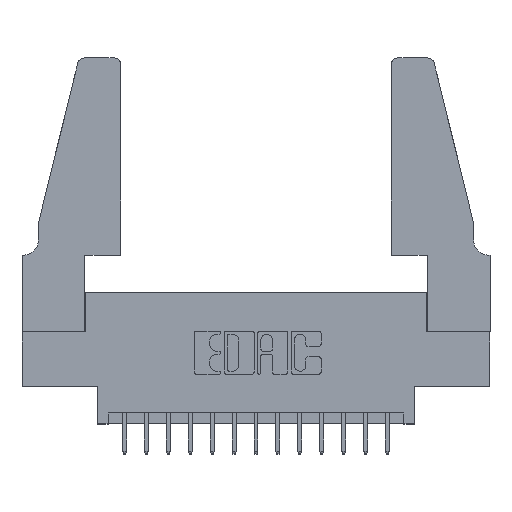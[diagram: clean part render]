
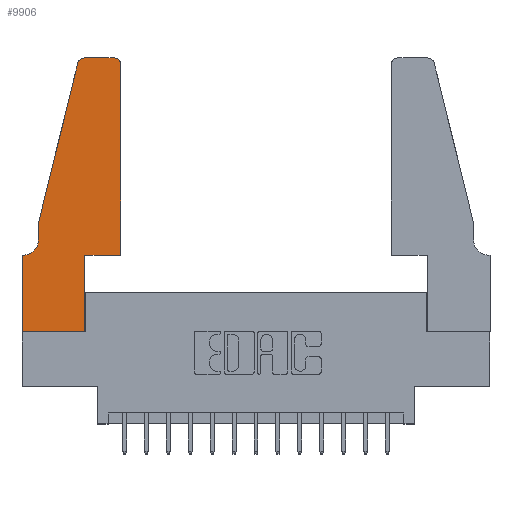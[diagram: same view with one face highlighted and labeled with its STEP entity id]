
A CAD part, top view. The second image highlights one B-rep face of the part: STEP entity #9906.
In plain terms, the highlighted planar face has unit normal (0, 0, 1).
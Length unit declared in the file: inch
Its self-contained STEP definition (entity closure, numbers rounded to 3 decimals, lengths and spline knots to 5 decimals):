
#67 = VERTEX_POINT ( 'NONE', #14824 ) ;
#144 = EDGE_CURVE ( 'NONE', #6721, #2338, #1736, .T. ) ;
#222 = VECTOR ( 'NONE', #10647, 39.37008 ) ;
#294 = VECTOR ( 'NONE', #14271, 39.37008 ) ;
#307 = CIRCLE ( 'NONE', #7475, 0.03 ) ;
#400 = AXIS2_PLACEMENT_3D ( 'NONE', #9724, #16011, #10734 ) ;
#455 = VECTOR ( 'NONE', #13324, 39.37008 ) ;
#547 = DIRECTION ( 'NONE',  ( 0., 0., 1. ) ) ;
#658 = FACE_OUTER_BOUND ( 'NONE', #4460, .T. ) ;
#707 = DIRECTION ( 'NONE',  ( 1., 0., 0. ) ) ;
#747 = ORIENTED_EDGE ( 'NONE', *, *, #5986, .T. ) ;
#981 = EDGE_CURVE ( 'NONE', #67, #6360, #307, .T. ) ;
#1228 = VECTOR ( 'NONE', #3764, 39.37008 ) ;
#1661 = CARTESIAN_POINT ( 'NONE',  ( 0.4505, 0.35, 0.37 ) ) ;
#1736 = LINE ( 'NONE', #14300, #1880 ) ;
#1793 = CARTESIAN_POINT ( 'NONE',  ( 0.4205, 1.22, 0.37 ) ) ;
#1880 = VECTOR ( 'NONE', #11884, 39.37008 ) ;
#1903 = ORIENTED_EDGE ( 'NONE', *, *, #981, .T. ) ;
#2084 = ORIENTED_EDGE ( 'NONE', *, *, #7525, .T. ) ;
#2115 = ORIENTED_EDGE ( 'NONE', *, *, #6188, .T. ) ;
#2148 = ORIENTED_EDGE ( 'NONE', *, *, #11866, .T. ) ;
#2187 = CARTESIAN_POINT ( 'NONE',  ( 0.0755, 0.42, 0.37 ) ) ;
#2338 = VERTEX_POINT ( 'NONE', #5541 ) ;
#2667 = LINE ( 'NONE', #5243, #4084 ) ;
#2964 = DIRECTION ( 'NONE',  ( 1., 0., 0. ) ) ;
#3192 = LINE ( 'NONE', #8264, #455 ) ;
#3261 = DIRECTION ( 'NONE',  ( 1., 0., 0. ) ) ;
#3445 = VECTOR ( 'NONE', #13188, 39.37008 ) ;
#3613 = CIRCLE ( 'NONE', #400, 0.07 ) ;
#3764 = DIRECTION ( 'NONE',  ( 1., 0., 0. ) ) ;
#3795 = CARTESIAN_POINT ( 'NONE',  ( 0.2865, 0.35, 0.37 ) ) ;
#4025 = LINE ( 'NONE', #1661, #222 ) ;
#4084 = VECTOR ( 'NONE', #5172, 39.37008 ) ;
#4460 = EDGE_LOOP ( 'NONE', ( #15340, #8765, #2148, #747, #7511, #15331, #2115, #14360, #8690, #2084, #14516, #1903 ) ) ;
#4502 = PLANE ( 'NONE',  #6140 ) ;
#5080 = AXIS2_PLACEMENT_3D ( 'NONE', #14353, #9366, #2964 ) ;
#5172 = DIRECTION ( 'NONE',  ( 0., 1., 0. ) ) ;
#5243 = CARTESIAN_POINT ( 'NONE',  ( 0.4505, 0.35, 0.37 ) ) ;
#5510 = VERTEX_POINT ( 'NONE', #11122 ) ;
#5523 = LINE ( 'NONE', #10587, #3445 ) ;
#5538 = CARTESIAN_POINT ( 'NONE',  ( 0.0755, 0.5, 0.37 ) ) ;
#5541 = CARTESIAN_POINT ( 'NONE',  ( 0., 0.35, 0.37 ) ) ;
#5585 = CARTESIAN_POINT ( 'NONE',  ( 0.4505, 0.35, 0.37 ) ) ;
#5857 = VERTEX_POINT ( 'NONE', #10749 ) ;
#5901 = EDGE_CURVE ( 'NONE', #11037, #12097, #3192, .T. ) ;
#5945 = EDGE_CURVE ( 'NONE', #6168, #11037, #12660, .T. ) ;
#5986 = EDGE_CURVE ( 'NONE', #5510, #6455, #7487, .T. ) ;
#6140 = AXIS2_PLACEMENT_3D ( 'NONE', #9565, #14644, #3261 ) ;
#6168 = VERTEX_POINT ( 'NONE', #11300 ) ;
#6188 = EDGE_CURVE ( 'NONE', #2338, #6168, #16323, .T. ) ;
#6360 = VERTEX_POINT ( 'NONE', #7280 ) ;
#6455 = VERTEX_POINT ( 'NONE', #2187 ) ;
#6721 = VERTEX_POINT ( 'NONE', #14178 ) ;
#7227 = EDGE_CURVE ( 'NONE', #6360, #9003, #5523, .T. ) ;
#7280 = CARTESIAN_POINT ( 'NONE',  ( 0.4205, 1.25, 0.37 ) ) ;
#7475 = AXIS2_PLACEMENT_3D ( 'NONE', #1793, #547, #707 ) ;
#7487 = LINE ( 'NONE', #7645, #11611 ) ;
#7511 = ORIENTED_EDGE ( 'NONE', *, *, #16413, .T. ) ;
#7525 = EDGE_CURVE ( 'NONE', #12097, #8520, #4025, .T. ) ;
#7645 = CARTESIAN_POINT ( 'NONE',  ( 0.0755, 0.5, 0.37 ) ) ;
#8206 = CARTESIAN_POINT ( 'NONE',  ( 0.284, 1.25, 0.37 ) ) ;
#8264 = CARTESIAN_POINT ( 'NONE',  ( 0.2865, 0.35, 0.37 ) ) ;
#8520 = VERTEX_POINT ( 'NONE', #5585 ) ;
#8522 = CIRCLE ( 'NONE', #5080, 0.03 ) ;
#8690 = ORIENTED_EDGE ( 'NONE', *, *, #5901, .T. ) ;
#8765 = ORIENTED_EDGE ( 'NONE', *, *, #11898, .T. ) ;
#9003 = VERTEX_POINT ( 'NONE', #8206 ) ;
#9366 = DIRECTION ( 'NONE',  ( 0., 0., 1. ) ) ;
#9444 = LINE ( 'NONE', #5538, #294 ) ;
#9565 = CARTESIAN_POINT ( 'NONE',  ( 0., 0.35, 0.37 ) ) ;
#9724 = CARTESIAN_POINT ( 'NONE',  ( 0.0055, 0.42, 0.37 ) ) ;
#9906 = ADVANCED_FACE ( 'NONE', ( #658 ), #4502, .T. ) ;
#10028 = DIRECTION ( 'NONE',  ( 0., -1., 0. ) ) ;
#10587 = CARTESIAN_POINT ( 'NONE',  ( 0.2605, 1.25, 0.37 ) ) ;
#10647 = DIRECTION ( 'NONE',  ( 1., 0., 0. ) ) ;
#10734 = DIRECTION ( 'NONE',  ( -1., 0., 0. ) ) ;
#10749 = CARTESIAN_POINT ( 'NONE',  ( 0.25487, 1.22718, 0.37 ) ) ;
#11037 = VERTEX_POINT ( 'NONE', #16328 ) ;
#11122 = CARTESIAN_POINT ( 'NONE',  ( 0.0755, 0.5, 0.37 ) ) ;
#11300 = CARTESIAN_POINT ( 'NONE',  ( 0., 0., 0.37 ) ) ;
#11611 = VECTOR ( 'NONE', #15338, 39.37008 ) ;
#11866 = EDGE_CURVE ( 'NONE', #5857, #5510, #9444, .T. ) ;
#11884 = DIRECTION ( 'NONE',  ( -1., 0., 0. ) ) ;
#11898 = EDGE_CURVE ( 'NONE', #9003, #5857, #8522, .T. ) ;
#12097 = VERTEX_POINT ( 'NONE', #3795 ) ;
#12115 = CARTESIAN_POINT ( 'NONE',  ( 0., 0., 0.37 ) ) ;
#12660 = LINE ( 'NONE', #12115, #1228 ) ;
#13188 = DIRECTION ( 'NONE',  ( -1., 0., 0. ) ) ;
#13324 = DIRECTION ( 'NONE',  ( 0., 1., 0. ) ) ;
#13689 = EDGE_CURVE ( 'NONE', #8520, #67, #2667, .T. ) ;
#13871 = CARTESIAN_POINT ( 'NONE',  ( 0., 0., 0.37 ) ) ;
#14178 = CARTESIAN_POINT ( 'NONE',  ( 0.0055, 0.35, 0.37 ) ) ;
#14271 = DIRECTION ( 'NONE',  ( -0.239, -0.971, 0. ) ) ;
#14300 = CARTESIAN_POINT ( 'NONE',  ( 0.0755, 0.35, 0.37 ) ) ;
#14353 = CARTESIAN_POINT ( 'NONE',  ( 0.284, 1.22, 0.37 ) ) ;
#14360 = ORIENTED_EDGE ( 'NONE', *, *, #5945, .T. ) ;
#14516 = ORIENTED_EDGE ( 'NONE', *, *, #13689, .T. ) ;
#14644 = DIRECTION ( 'NONE',  ( 0., 0., 1. ) ) ;
#14824 = CARTESIAN_POINT ( 'NONE',  ( 0.4505, 1.22, 0.37 ) ) ;
#15331 = ORIENTED_EDGE ( 'NONE', *, *, #144, .T. ) ;
#15338 = DIRECTION ( 'NONE',  ( 0., -1., 0. ) ) ;
#15340 = ORIENTED_EDGE ( 'NONE', *, *, #7227, .T. ) ;
#15924 = VECTOR ( 'NONE', #10028, 39.37008 ) ;
#16011 = DIRECTION ( 'NONE',  ( 0., 0., -1. ) ) ;
#16323 = LINE ( 'NONE', #13871, #15924 ) ;
#16328 = CARTESIAN_POINT ( 'NONE',  ( 0.2865, 0., 0.37 ) ) ;
#16413 = EDGE_CURVE ( 'NONE', #6455, #6721, #3613, .T. ) ;
